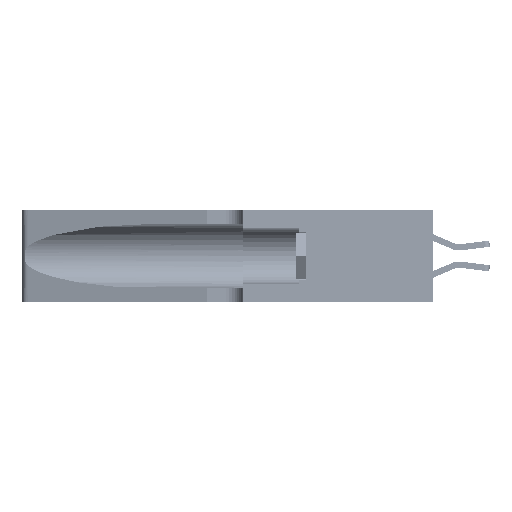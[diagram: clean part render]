
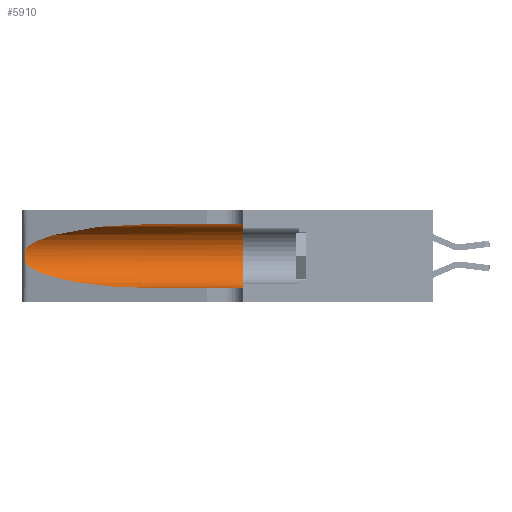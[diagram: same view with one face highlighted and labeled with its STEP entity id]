
A CAD part, left-side view. The second image highlights one B-rep face of the part: STEP entity #5910.
In plain terms, the highlighted cylindrical face has radius 3.308 mm (diameter 6.617 mm), a partial arc.
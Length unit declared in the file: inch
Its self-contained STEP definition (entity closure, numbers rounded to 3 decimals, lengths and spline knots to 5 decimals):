
#1713 =( BOUNDED_CURVE ( )  B_SPLINE_CURVE ( 3, ( #39208, #34841, #12728, #31616 ),
 .UNSPECIFIED., .F., .F. ) 
 B_SPLINE_CURVE_WITH_KNOTS ( ( 4, 4 ),
 ( 3.44316, 4.71239 ),
 .UNSPECIFIED. ) 
 CURVE ( )  GEOMETRIC_REPRESENTATION_ITEM ( )  RATIONAL_B_SPLINE_CURVE ( ( 1., 0.87, 0.87, 1. ) ) 
 REPRESENTATION_ITEM ( '' )  );
#4749 = CARTESIAN_POINT ( 'NONE',  ( 0.1305, 0.35, 0.31525 ) ) ;
#5192 = ORIENTED_EDGE ( 'NONE', *, *, #34285, .T. ) ;
#5910 = ADVANCED_FACE ( 'NONE', ( #33767 ), #32027, .F. ) ;
#7122 = DIRECTION ( 'NONE',  ( 0., 0., -1. ) ) ;
#9627 = CARTESIAN_POINT ( 'NONE',  ( 0.1305, 1.61858, 0.31525 ) ) ;
#9775 = DIRECTION ( 'NONE',  ( 0., -1., 0. ) ) ;
#10037 = VERTEX_POINT ( 'NONE', #14605 ) ;
#10464 = CARTESIAN_POINT ( 'NONE',  ( 0.1305, 0.72297, 0.31525 ) ) ;
#12544 = CARTESIAN_POINT ( 'NONE',  ( 0.25787, 1.23484, 0.2124 ) ) ;
#12714 = B_SPLINE_CURVE_WITH_KNOTS ( 'NONE', 3,
 ( #16376, #34500, #45685, #12544, #42091, #23465, #38386, #19902, #16529, #42564, #23764, #20060, #27653, #20363 ),
 .UNSPECIFIED., .F., .F.,
 ( 4, 2, 2, 2, 2, 2, 4 ),
 ( 0., 0.00027, 0.00053, 0.00107, 0.0016, 0.00187, 0.00214 ),
 .UNSPECIFIED. ) ;
#12728 = CARTESIAN_POINT ( 'NONE',  ( 0.18966, 0.96281, 0.05475 ) ) ;
#13595 = EDGE_CURVE ( 'NONE', #37887, #23746, #32802, .T. ) ;
#13752 = CARTESIAN_POINT ( 'NONE',  ( 0.1305, 1.61858, 0.185 ) ) ;
#14605 = CARTESIAN_POINT ( 'NONE',  ( 0.1305, 0.35, 0.05475 ) ) ;
#16376 = CARTESIAN_POINT ( 'NONE',  ( 0.25487, 1.22718, 0.22369 ) ) ;
#16529 = CARTESIAN_POINT ( 'NONE',  ( 0.26017, 1.23833, 0.17102 ) ) ;
#17123 = ORIENTED_EDGE ( 'NONE', *, *, #47055, .T. ) ;
#19902 = CARTESIAN_POINT ( 'NONE',  ( 0.26075, 1.23896, 0.178 ) ) ;
#20060 = CARTESIAN_POINT ( 'NONE',  ( 0.25639, 1.23186, 0.15144 ) ) ;
#20363 = CARTESIAN_POINT ( 'NONE',  ( 0.25487, 1.22718, 0.14631 ) ) ;
#21833 = CARTESIAN_POINT ( 'NONE',  ( 0.2373, 1.15595, 0.28018 ) ) ;
#23465 = CARTESIAN_POINT ( 'NONE',  ( 0.26018, 1.23835, 0.19895 ) ) ;
#23746 = VERTEX_POINT ( 'NONE', #4749 ) ;
#23764 = CARTESIAN_POINT ( 'NONE',  ( 0.25789, 1.23486, 0.15765 ) ) ;
#23956 = VERTEX_POINT ( 'NONE', #35435 ) ;
#24962 = LINE ( 'NONE', #28458, #38294 ) ;
#25675 = ORIENTED_EDGE ( 'NONE', *, *, #27399, .T. ) ;
#26402 = VECTOR ( 'NONE', #43358, 39.37008 ) ;
#27135 = DIRECTION ( 'NONE',  ( 0., 1., 0. ) ) ;
#27399 = EDGE_CURVE ( 'NONE', #37126, #10037, #24962, .T. ) ;
#27653 = CARTESIAN_POINT ( 'NONE',  ( 0.25555, 1.22993, 0.14849 ) ) ;
#27930 = AXIS2_PLACEMENT_3D ( 'NONE', #30253, #27135, #45492 ) ;
#28458 = CARTESIAN_POINT ( 'NONE',  ( 0.1305, 1.61858, 0.05475 ) ) ;
#30253 = CARTESIAN_POINT ( 'NONE',  ( 0.1305, 0.35, 0.185 ) ) ;
#30955 = EDGE_CURVE ( 'NONE', #23956, #34355, #12714, .T. ) ;
#31112 = ORIENTED_EDGE ( 'NONE', *, *, #13595, .F. ) ;
#31281 = ORIENTED_EDGE ( 'NONE', *, *, #30955, .T. ) ;
#31616 = CARTESIAN_POINT ( 'NONE',  ( 0.1305, 0.72297, 0.05475 ) ) ;
#32027 = CYLINDRICAL_SURFACE ( 'NONE', #46384, 0.13025 ) ;
#32255 = DIRECTION ( 'NONE',  ( 0., -1., 0. ) ) ;
#32802 = LINE ( 'NONE', #9627, #26402 ) ;
#33159 = ORIENTED_EDGE ( 'NONE', *, *, #34571, .F. ) ;
#33767 = FACE_OUTER_BOUND ( 'NONE', #39482, .T. ) ;
#34285 = EDGE_CURVE ( 'NONE', #37887, #23956, #43499, .T. ) ;
#34355 = VERTEX_POINT ( 'NONE', #37215 ) ;
#34500 = CARTESIAN_POINT ( 'NONE',  ( 0.25555, 1.22994, 0.2215 ) ) ;
#34571 = EDGE_CURVE ( 'NONE', #23746, #10037, #37161, .T. ) ;
#34841 = CARTESIAN_POINT ( 'NONE',  ( 0.2373, 1.15595, 0.08982 ) ) ;
#35435 = CARTESIAN_POINT ( 'NONE',  ( 0.25487, 1.22718, 0.22369 ) ) ;
#35549 = CARTESIAN_POINT ( 'NONE',  ( 0.1305, 0.72297, 0.31525 ) ) ;
#37126 = VERTEX_POINT ( 'NONE', #46312 ) ;
#37161 = CIRCLE ( 'NONE', #27930, 0.13025 ) ;
#37215 = CARTESIAN_POINT ( 'NONE',  ( 0.25487, 1.22718, 0.14631 ) ) ;
#37887 = VERTEX_POINT ( 'NONE', #35549 ) ;
#38294 = VECTOR ( 'NONE', #32255, 39.37008 ) ;
#38386 = CARTESIAN_POINT ( 'NONE',  ( 0.26075, 1.23896, 0.19203 ) ) ;
#39208 = CARTESIAN_POINT ( 'NONE',  ( 0.25487, 1.22718, 0.14631 ) ) ;
#39482 = EDGE_LOOP ( 'NONE', ( #5192, #31281, #17123, #25675, #33159, #31112 ) ) ;
#40475 = CARTESIAN_POINT ( 'NONE',  ( 0.18966, 0.96281, 0.31525 ) ) ;
#42091 = CARTESIAN_POINT ( 'NONE',  ( 0.25854, 1.2359, 0.20912 ) ) ;
#42564 = CARTESIAN_POINT ( 'NONE',  ( 0.25856, 1.23593, 0.16098 ) ) ;
#43358 = DIRECTION ( 'NONE',  ( 0., -1., 0. ) ) ;
#43499 =( BOUNDED_CURVE ( )  B_SPLINE_CURVE ( 3, ( #10464, #40475, #21833, #47289 ),
 .UNSPECIFIED., .F., .T. ) 
 B_SPLINE_CURVE_WITH_KNOTS ( ( 4, 4 ),
 ( 1.5708, 2.84003 ),
 .UNSPECIFIED. ) 
 CURVE ( )  GEOMETRIC_REPRESENTATION_ITEM ( )  RATIONAL_B_SPLINE_CURVE ( ( 1., 0.87, 0.87, 1. ) ) 
 REPRESENTATION_ITEM ( '' )  );
#45492 = DIRECTION ( 'NONE',  ( 0., 0., 1. ) ) ;
#45685 = CARTESIAN_POINT ( 'NONE',  ( 0.25639, 1.23184, 0.21858 ) ) ;
#46312 = CARTESIAN_POINT ( 'NONE',  ( 0.1305, 0.72297, 0.05475 ) ) ;
#46384 = AXIS2_PLACEMENT_3D ( 'NONE', #13752, #9775, #7122 ) ;
#47055 = EDGE_CURVE ( 'NONE', #34355, #37126, #1713, .T. ) ;
#47289 = CARTESIAN_POINT ( 'NONE',  ( 0.25487, 1.22718, 0.22369 ) ) ;
